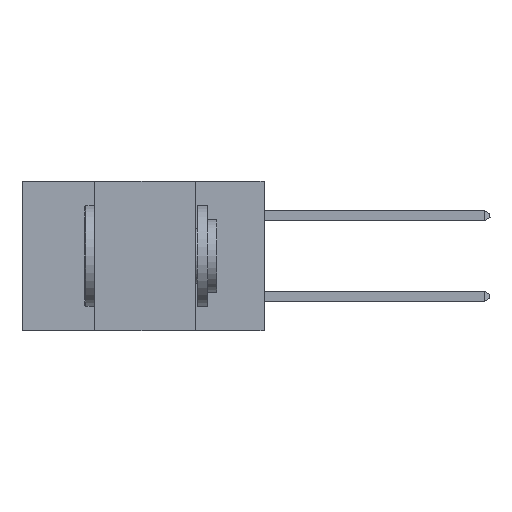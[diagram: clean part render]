
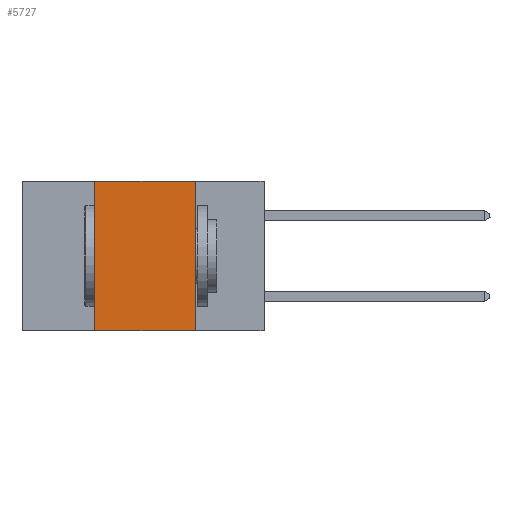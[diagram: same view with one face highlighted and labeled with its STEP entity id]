
A CAD part, left-side view. The second image highlights one B-rep face of the part: STEP entity #5727.
In plain terms, the highlighted planar face has unit normal (-1, 0, 0).
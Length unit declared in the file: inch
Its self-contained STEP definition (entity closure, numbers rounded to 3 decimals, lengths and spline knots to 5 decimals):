
#424 = LINE ( 'NONE', #18440, #8094 ) ;
#631 = VECTOR ( 'NONE', #13532, 39.37008 ) ;
#996 = VERTEX_POINT ( 'NONE', #11441 ) ;
#1146 = CARTESIAN_POINT ( 'NONE',  ( 0., 0.6, -0.37 ) ) ;
#1743 = CARTESIAN_POINT ( 'NONE',  ( 0., 0.17, -0.37 ) ) ;
#2527 = EDGE_CURVE ( 'NONE', #22783, #8430, #3134, .T. ) ;
#3134 = LINE ( 'NONE', #14921, #21429 ) ;
#3287 = CARTESIAN_POINT ( 'NONE',  ( 0., 0.6, 0. ) ) ;
#3638 = ORIENTED_EDGE ( 'NONE', *, *, #2527, .F. ) ;
#4158 = ORIENTED_EDGE ( 'NONE', *, *, #9630, .F. ) ;
#5161 = ORIENTED_EDGE ( 'NONE', *, *, #16184, .T. ) ;
#5727 = ADVANCED_FACE ( 'NONE', ( #27551 ), #11960, .F. ) ;
#7442 = ORIENTED_EDGE ( 'NONE', *, *, #12818, .F. ) ;
#7503 = DIRECTION ( 'NONE',  ( 1., 0., 0. ) ) ;
#8094 = VECTOR ( 'NONE', #26465, 39.37008 ) ;
#8162 = VERTEX_POINT ( 'NONE', #16126 ) ;
#8430 = VERTEX_POINT ( 'NONE', #1743 ) ;
#9630 = EDGE_CURVE ( 'NONE', #996, #8162, #22891, .T. ) ;
#10522 = VECTOR ( 'NONE', #12067, 39.37008 ) ;
#11441 = CARTESIAN_POINT ( 'NONE',  ( 0., 0.42, -0.37 ) ) ;
#11960 = PLANE ( 'NONE',  #15615 ) ;
#12067 = DIRECTION ( 'NONE',  ( 0., -1., 0. ) ) ;
#12818 = EDGE_CURVE ( 'NONE', #8162, #22783, #424, .T. ) ;
#13532 = DIRECTION ( 'NONE',  ( 0., 0., 1. ) ) ;
#14921 = CARTESIAN_POINT ( 'NONE',  ( 0., 0.17, 0. ) ) ;
#15615 = AXIS2_PLACEMENT_3D ( 'NONE', #3287, #7503, #22147 ) ;
#16126 = CARTESIAN_POINT ( 'NONE',  ( 0., 0.42, 0. ) ) ;
#16184 = EDGE_CURVE ( 'NONE', #996, #8430, #17238, .T. ) ;
#17238 = LINE ( 'NONE', #1146, #10522 ) ;
#17829 = CARTESIAN_POINT ( 'NONE',  ( 0., 0.42, 0. ) ) ;
#18440 = CARTESIAN_POINT ( 'NONE',  ( 0., 0.6, 0. ) ) ;
#19490 = EDGE_LOOP ( 'NONE', ( #3638, #7442, #4158, #5161 ) ) ;
#21281 = DIRECTION ( 'NONE',  ( 0., 0., -1. ) ) ;
#21429 = VECTOR ( 'NONE', #21281, 39.37008 ) ;
#22147 = DIRECTION ( 'NONE',  ( 0., 0., -1. ) ) ;
#22647 = CARTESIAN_POINT ( 'NONE',  ( 0., 0.17, 0. ) ) ;
#22783 = VERTEX_POINT ( 'NONE', #22647 ) ;
#22891 = LINE ( 'NONE', #17829, #631 ) ;
#26465 = DIRECTION ( 'NONE',  ( 0., -1., 0. ) ) ;
#27551 = FACE_OUTER_BOUND ( 'NONE', #19490, .T. ) ;
